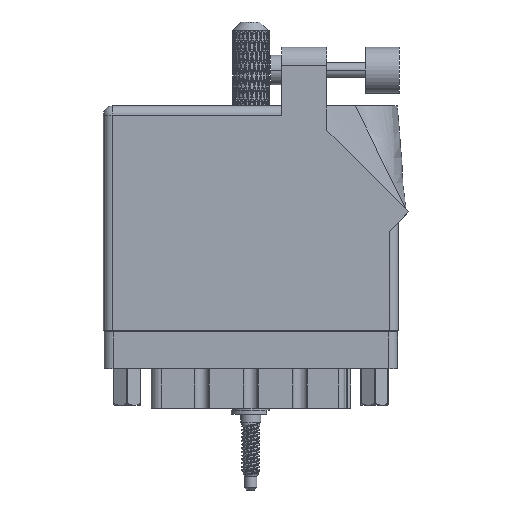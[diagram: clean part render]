
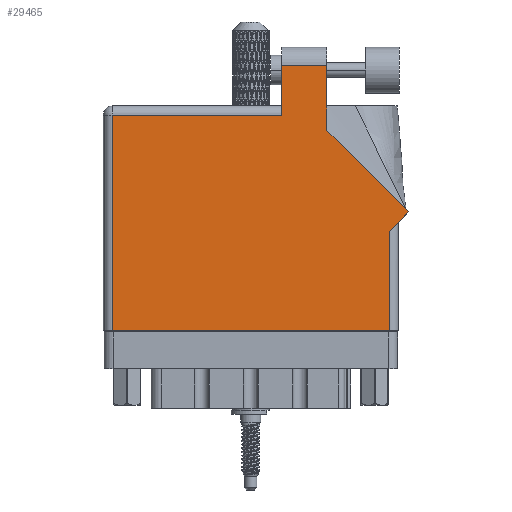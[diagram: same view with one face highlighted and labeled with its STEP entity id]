
A CAD part, front view. The second image highlights one B-rep face of the part: STEP entity #29465.
In plain terms, the highlighted face is planar.
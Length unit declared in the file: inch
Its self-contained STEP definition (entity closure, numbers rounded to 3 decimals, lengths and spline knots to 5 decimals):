
#747 = DIRECTION ( 'NONE',  ( 0., 0., -1. ) ) ;
#1541 = CARTESIAN_POINT ( 'NONE',  ( 1.524, 1.805, 0. ) ) ;
#2130 = CARTESIAN_POINT ( 'NONE',  ( 1.217, 1.805, 0. ) ) ;
#2296 = VECTOR ( 'NONE', #74707, 39.37008 ) ;
#2746 = CARTESIAN_POINT ( 'NONE',  ( 2.08071, 0.80771, 0. ) ) ;
#2986 = ORIENTED_EDGE ( 'NONE', *, *, #60158, .T. ) ;
#5026 = VERTEX_POINT ( 'NONE', #23059 ) ;
#7294 = ORIENTED_EDGE ( 'NONE', *, *, #37028, .T. ) ;
#7682 = LINE ( 'NONE', #22466, #76232 ) ;
#9056 = LINE ( 'NONE', #14541, #24408 ) ;
#9665 = EDGE_CURVE ( 'NONE', #63085, #50478, #85096, .T. ) ;
#11700 = CARTESIAN_POINT ( 'NONE',  ( 0., 1.468, 0. ) ) ;
#12984 = CARTESIAN_POINT ( 'NONE',  ( 0.062, 1.468, 0. ) ) ;
#13275 = DIRECTION ( 'NONE',  ( -0.707, 0.707, 0. ) ) ;
#14347 = EDGE_CURVE ( 'NONE', #78413, #63085, #18409, .T. ) ;
#14541 = CARTESIAN_POINT ( 'NONE',  ( 1.217, 1.805, 0. ) ) ;
#14918 = DIRECTION ( 'NONE',  ( -1., 0., 0. ) ) ;
#17809 = FACE_OUTER_BOUND ( 'NONE', #24656, .T. ) ;
#18409 = LINE ( 'NONE', #33763, #95343 ) ;
#19271 = EDGE_CURVE ( 'NONE', #5026, #36601, #51258, .T. ) ;
#20029 = AXIS2_PLACEMENT_3D ( 'NONE', #89087, #747, #80125 ) ;
#21107 = CARTESIAN_POINT ( 'NONE',  ( 1.524, 1.36442, 0. ) ) ;
#22466 = CARTESIAN_POINT ( 'NONE',  ( 1.948, 0.737, 0. ) ) ;
#23059 = CARTESIAN_POINT ( 'NONE',  ( 0.062, 0., 0. ) ) ;
#23166 = ORIENTED_EDGE ( 'NONE', *, *, #82426, .T. ) ;
#24408 = VECTOR ( 'NONE', #14918, 39.37008 ) ;
#24656 = EDGE_LOOP ( 'NONE', ( #42448, #68509, #25428, #89121, #7294, #63344, #23166, #35119, #2986 ) ) ;
#25428 = ORIENTED_EDGE ( 'NONE', *, *, #14347, .T. ) ;
#26552 = CARTESIAN_POINT ( 'NONE',  ( 1.948, 0.675, 0. ) ) ;
#28933 = VERTEX_POINT ( 'NONE', #29491 ) ;
#29465 = ADVANCED_FACE ( 'NONE', ( #17809 ), #71095, .F. ) ;
#29491 = CARTESIAN_POINT ( 'NONE',  ( 2.08071, 0.80771, 0. ) ) ;
#31878 = VERTEX_POINT ( 'NONE', #1541 ) ;
#32683 = DIRECTION ( 'NONE',  ( 0., 1., 0. ) ) ;
#33763 = CARTESIAN_POINT ( 'NONE',  ( 1.217, 1.53, 0. ) ) ;
#35119 = ORIENTED_EDGE ( 'NONE', *, *, #88643, .T. ) ;
#35714 = CARTESIAN_POINT ( 'NONE',  ( 0.062, 0., 0. ) ) ;
#36601 = VERTEX_POINT ( 'NONE', #102986 ) ;
#37028 = EDGE_CURVE ( 'NONE', #50478, #5026, #75927, .T. ) ;
#38969 = VECTOR ( 'NONE', #75001, 39.37008 ) ;
#41372 = LINE ( 'NONE', #2746, #97291 ) ;
#42448 = ORIENTED_EDGE ( 'NONE', *, *, #80913, .T. ) ;
#47127 = VECTOR ( 'NONE', #76326, 39.37008 ) ;
#50478 = VERTEX_POINT ( 'NONE', #12984 ) ;
#50780 = VECTOR ( 'NONE', #114165, 39.37008 ) ;
#51258 = LINE ( 'NONE', #57595, #47127 ) ;
#55465 = LINE ( 'NONE', #21107, #2296 ) ;
#57540 = VECTOR ( 'NONE', #81276, 39.37008 ) ;
#57595 = CARTESIAN_POINT ( 'NONE',  ( 0., 0., 0. ) ) ;
#60158 = EDGE_CURVE ( 'NONE', #28933, #99794, #41372, .T. ) ;
#61272 = VERTEX_POINT ( 'NONE', #26552 ) ;
#63085 = VERTEX_POINT ( 'NONE', #71591 ) ;
#63344 = ORIENTED_EDGE ( 'NONE', *, *, #19271, .T. ) ;
#68509 = ORIENTED_EDGE ( 'NONE', *, *, #90191, .T. ) ;
#70188 = LINE ( 'NONE', #89861, #57540 ) ;
#71095 = PLANE ( 'NONE',  #20029 ) ;
#71591 = CARTESIAN_POINT ( 'NONE',  ( 1.217, 1.468, 0. ) ) ;
#74707 = DIRECTION ( 'NONE',  ( 0., 1., 0. ) ) ;
#75001 = DIRECTION ( 'NONE',  ( -1., 0., 0. ) ) ;
#75927 = LINE ( 'NONE', #35714, #50780 ) ;
#76232 = VECTOR ( 'NONE', #32683, 39.37008 ) ;
#76326 = DIRECTION ( 'NONE',  ( 1., 0., 0. ) ) ;
#77883 = DIRECTION ( 'NONE',  ( 0., -1., 0. ) ) ;
#78413 = VERTEX_POINT ( 'NONE', #2130 ) ;
#80125 = DIRECTION ( 'NONE',  ( -1., 0., 0. ) ) ;
#80913 = EDGE_CURVE ( 'NONE', #99794, #31878, #55465, .T. ) ;
#81276 = DIRECTION ( 'NONE',  ( 0.707, 0.707, 0. ) ) ;
#82426 = EDGE_CURVE ( 'NONE', #36601, #61272, #7682, .T. ) ;
#85096 = LINE ( 'NONE', #11700, #38969 ) ;
#85560 = CARTESIAN_POINT ( 'NONE',  ( 1.524, 1.36442, 0. ) ) ;
#88643 = EDGE_CURVE ( 'NONE', #61272, #28933, #70188, .T. ) ;
#89087 = CARTESIAN_POINT ( 'NONE',  ( 0., 1.53, 0. ) ) ;
#89121 = ORIENTED_EDGE ( 'NONE', *, *, #9665, .T. ) ;
#89861 = CARTESIAN_POINT ( 'NONE',  ( 2.01, 0.737, 0. ) ) ;
#90191 = EDGE_CURVE ( 'NONE', #31878, #78413, #9056, .T. ) ;
#95343 = VECTOR ( 'NONE', #77883, 39.37008 ) ;
#97291 = VECTOR ( 'NONE', #13275, 39.37008 ) ;
#99794 = VERTEX_POINT ( 'NONE', #85560 ) ;
#102986 = CARTESIAN_POINT ( 'NONE',  ( 1.948, 0., 0. ) ) ;
#114165 = DIRECTION ( 'NONE',  ( 0., -1., 0. ) ) ;
